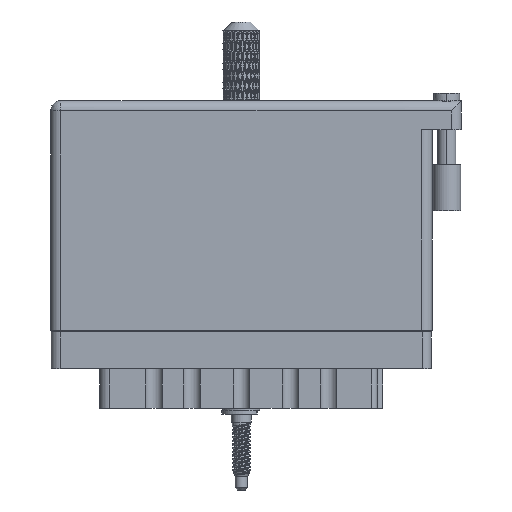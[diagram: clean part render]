
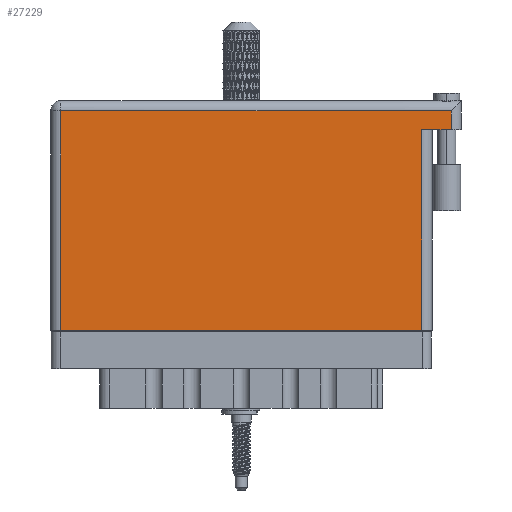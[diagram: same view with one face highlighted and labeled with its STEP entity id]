
A CAD part, front view. The second image highlights one B-rep face of the part: STEP entity #27229.
In plain terms, the highlighted face is planar.
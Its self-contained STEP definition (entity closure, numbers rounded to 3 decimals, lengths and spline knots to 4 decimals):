
#2257 = CARTESIAN_POINT ( 'NONE',  ( 2.8, 1.369, 0. ) ) ;
#2358 = VECTOR ( 'NONE', #48170, 39.3701 ) ;
#5145 = VECTOR ( 'NONE', #52743, 39.3701 ) ;
#5319 = CARTESIAN_POINT ( 'NONE',  ( 2.73, 1.566, 0. ) ) ;
#9305 = LINE ( 'NONE', #2257, #12211 ) ;
#12211 = VECTOR ( 'NONE', #111918, 39.3701 ) ;
#12314 = LINE ( 'NONE', #5319, #5145 ) ;
#13561 = CARTESIAN_POINT ( 'NONE',  ( 0.07, 1.496, 0. ) ) ;
#13804 = CARTESIAN_POINT ( 'NONE',  ( 2.73, 1.369, 0. ) ) ;
#15606 = PLANE ( 'NONE',  #107728 ) ;
#15956 = VERTEX_POINT ( 'NONE', #13561 ) ;
#18940 = DIRECTION ( 'NONE',  ( 1., 0., 0. ) ) ;
#22148 = DIRECTION ( 'NONE',  ( -1., 0., 0. ) ) ;
#26142 = LINE ( 'NONE', #111269, #59225 ) ;
#26571 = VERTEX_POINT ( 'NONE', #82968 ) ;
#27229 = ADVANCED_FACE ( 'NONE', ( #67158 ), #15606, .F. ) ;
#29195 = CARTESIAN_POINT ( 'NONE',  ( 2.73, 1.496, 0. ) ) ;
#30636 = EDGE_LOOP ( 'NONE', ( #57422, #108495, #94382, #91375, #61403, #33550 ) ) ;
#32228 = VECTOR ( 'NONE', #22148, 39.3701 ) ;
#33550 = ORIENTED_EDGE ( 'NONE', *, *, #104782, .T. ) ;
#34084 = DIRECTION ( 'NONE',  ( 0., 0., -1. ) ) ;
#42235 = CARTESIAN_POINT ( 'NONE',  ( 2.53, 1.369, 0. ) ) ;
#47766 = CARTESIAN_POINT ( 'NONE',  ( 2.53, 1.369, 0. ) ) ;
#48170 = DIRECTION ( 'NONE',  ( 0., 1., 0. ) ) ;
#52743 = DIRECTION ( 'NONE',  ( 0., 1., 0. ) ) ;
#55483 = CARTESIAN_POINT ( 'NONE',  ( 0., 0., 0. ) ) ;
#56649 = CARTESIAN_POINT ( 'NONE',  ( 2.53, 0., 0. ) ) ;
#57422 = ORIENTED_EDGE ( 'NONE', *, *, #111707, .T. ) ;
#59225 = VECTOR ( 'NONE', #101649, 39.3701 ) ;
#61403 = ORIENTED_EDGE ( 'NONE', *, *, #71170, .T. ) ;
#66564 = VERTEX_POINT ( 'NONE', #42235 ) ;
#67158 = FACE_OUTER_BOUND ( 'NONE', #30636, .T. ) ;
#67663 = VERTEX_POINT ( 'NONE', #56649 ) ;
#71170 = EDGE_CURVE ( 'NONE', #102921, #15956, #101164, .T. ) ;
#78056 = VERTEX_POINT ( 'NONE', #13804 ) ;
#79915 = CARTESIAN_POINT ( 'NONE',  ( 0., 1.566, 0. ) ) ;
#82968 = CARTESIAN_POINT ( 'NONE',  ( 0.07, 0., 0. ) ) ;
#86921 = VECTOR ( 'NONE', #18940, 39.3701 ) ;
#91375 = ORIENTED_EDGE ( 'NONE', *, *, #110402, .T. ) ;
#91535 = LINE ( 'NONE', #47766, #2358 ) ;
#94382 = ORIENTED_EDGE ( 'NONE', *, *, #112198, .F. ) ;
#96042 = CARTESIAN_POINT ( 'NONE',  ( 0., 1.496, 0. ) ) ;
#98397 = DIRECTION ( 'NONE',  ( -1., 0., 0. ) ) ;
#100673 = EDGE_CURVE ( 'NONE', #67663, #66564, #91535, .T. ) ;
#101164 = LINE ( 'NONE', #96042, #32228 ) ;
#101649 = DIRECTION ( 'NONE',  ( 0., -1., 0. ) ) ;
#102921 = VERTEX_POINT ( 'NONE', #29195 ) ;
#104782 = EDGE_CURVE ( 'NONE', #15956, #26571, #26142, .T. ) ;
#107728 = AXIS2_PLACEMENT_3D ( 'NONE', #79915, #34084, #98397 ) ;
#108495 = ORIENTED_EDGE ( 'NONE', *, *, #100673, .T. ) ;
#110402 = EDGE_CURVE ( 'NONE', #78056, #102921, #12314, .T. ) ;
#111269 = CARTESIAN_POINT ( 'NONE',  ( 0.07, 0., 0. ) ) ;
#111707 = EDGE_CURVE ( 'NONE', #26571, #67663, #117085, .T. ) ;
#111918 = DIRECTION ( 'NONE',  ( -1., 0., 0. ) ) ;
#112198 = EDGE_CURVE ( 'NONE', #78056, #66564, #9305, .T. ) ;
#117085 = LINE ( 'NONE', #55483, #86921 ) ;
